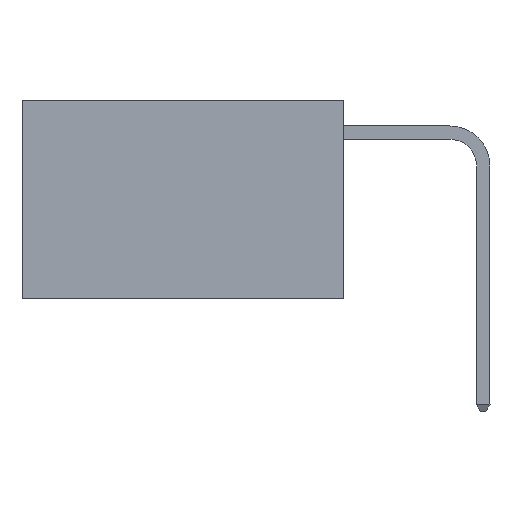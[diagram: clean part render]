
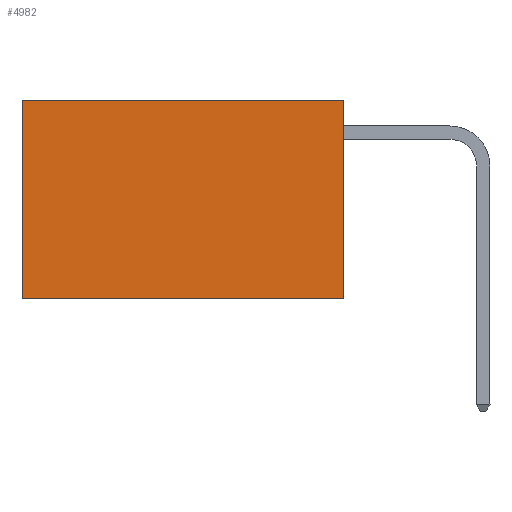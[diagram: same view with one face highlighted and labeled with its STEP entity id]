
A CAD part, left-side view. The second image highlights one B-rep face of the part: STEP entity #4982.
In plain terms, the highlighted planar face has unit normal (-1, 0, 0).
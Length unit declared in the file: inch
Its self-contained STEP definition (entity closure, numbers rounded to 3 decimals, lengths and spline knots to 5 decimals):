
#496 = VECTOR ( 'NONE', #623, 39.37008 ) ;
#623 = DIRECTION ( 'NONE',  ( 0., 1., 0. ) ) ;
#902 = EDGE_LOOP ( 'NONE', ( #8210, #4135, #5995, #4866 ) ) ;
#903 = VERTEX_POINT ( 'NONE', #4042 ) ;
#1741 = EDGE_CURVE ( 'NONE', #5993, #903, #7213, .T. ) ;
#2677 = LINE ( 'NONE', #7896, #496 ) ;
#2985 = VECTOR ( 'NONE', #6928, 39.37008 ) ;
#2991 = CARTESIAN_POINT ( 'NONE',  ( 0.2625, 0.6, 0. ) ) ;
#3304 = FACE_OUTER_BOUND ( 'NONE', #902, .T. ) ;
#3468 = EDGE_CURVE ( 'NONE', #4977, #7961, #8480, .T. ) ;
#3619 = CARTESIAN_POINT ( 'NONE',  ( 0.2625, 0., 0. ) ) ;
#4042 = CARTESIAN_POINT ( 'NONE',  ( 0.2625, 0., -0.37 ) ) ;
#4104 = VECTOR ( 'NONE', #4453, 39.37008 ) ;
#4135 = ORIENTED_EDGE ( 'NONE', *, *, #5438, .F. ) ;
#4424 = DIRECTION ( 'NONE',  ( 0., 0., -1. ) ) ;
#4453 = DIRECTION ( 'NONE',  ( 0., 1., 0. ) ) ;
#4755 = CARTESIAN_POINT ( 'NONE',  ( 0.2625, 0.6, -0.37 ) ) ;
#4866 = ORIENTED_EDGE ( 'NONE', *, *, #7419, .T. ) ;
#4977 = VERTEX_POINT ( 'NONE', #2991 ) ;
#4982 = ADVANCED_FACE ( 'NONE', ( #3304 ), #7968, .F. ) ;
#5111 = AXIS2_PLACEMENT_3D ( 'NONE', #3619, #8615, #4424 ) ;
#5438 = EDGE_CURVE ( 'NONE', #903, #7961, #8148, .T. ) ;
#5506 = VECTOR ( 'NONE', #7905, 39.37008 ) ;
#5983 = CARTESIAN_POINT ( 'NONE',  ( 0.2625, 0., 0. ) ) ;
#5993 = VERTEX_POINT ( 'NONE', #9177 ) ;
#5995 = ORIENTED_EDGE ( 'NONE', *, *, #1741, .F. ) ;
#6166 = CARTESIAN_POINT ( 'NONE',  ( 0.2625, 0.6, 0. ) ) ;
#6928 = DIRECTION ( 'NONE',  ( 0., 0., -1. ) ) ;
#7213 = LINE ( 'NONE', #5983, #5506 ) ;
#7305 = CARTESIAN_POINT ( 'NONE',  ( 0.2625, 0., -0.37 ) ) ;
#7419 = EDGE_CURVE ( 'NONE', #5993, #4977, #2677, .T. ) ;
#7896 = CARTESIAN_POINT ( 'NONE',  ( 0.2625, 0., 0. ) ) ;
#7905 = DIRECTION ( 'NONE',  ( 0., 0., -1. ) ) ;
#7961 = VERTEX_POINT ( 'NONE', #4755 ) ;
#7968 = PLANE ( 'NONE',  #5111 ) ;
#8148 = LINE ( 'NONE', #7305, #4104 ) ;
#8210 = ORIENTED_EDGE ( 'NONE', *, *, #3468, .T. ) ;
#8480 = LINE ( 'NONE', #6166, #2985 ) ;
#8615 = DIRECTION ( 'NONE',  ( 1., 0., 0. ) ) ;
#9177 = CARTESIAN_POINT ( 'NONE',  ( 0.2625, 0., 0. ) ) ;
